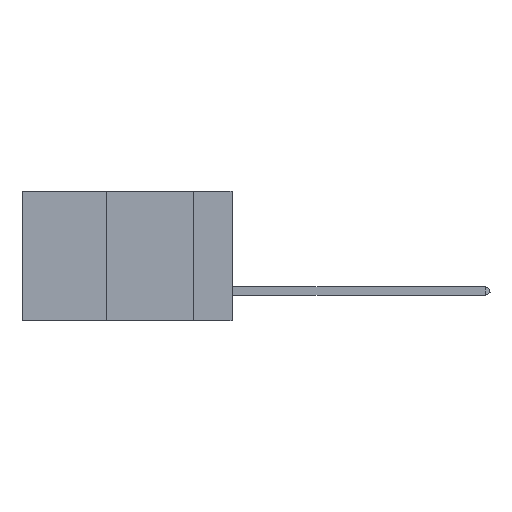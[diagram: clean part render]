
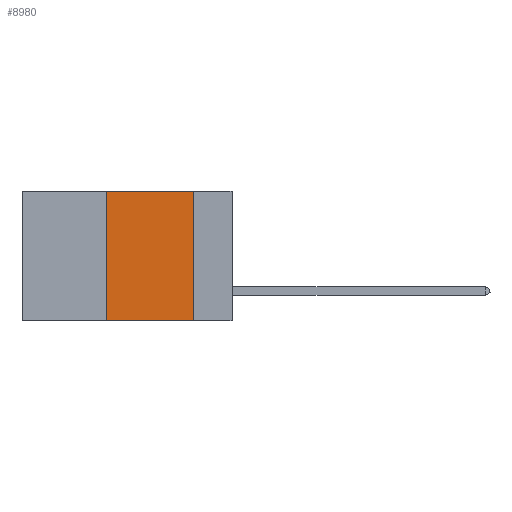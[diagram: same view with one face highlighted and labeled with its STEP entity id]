
A CAD part, left-side view. The second image highlights one B-rep face of the part: STEP entity #8980.
In plain terms, the highlighted planar face has unit normal (-1, 0, 0).
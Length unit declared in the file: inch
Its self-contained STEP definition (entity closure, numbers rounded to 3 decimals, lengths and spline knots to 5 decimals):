
#90 = VERTEX_POINT ( 'NONE', #13206 ) ;
#434 = CARTESIAN_POINT ( 'NONE',  ( 0., 0.6, -0.37 ) ) ;
#2119 = VECTOR ( 'NONE', #6401, 39.37008 ) ;
#2528 = VECTOR ( 'NONE', #12863, 39.37008 ) ;
#2623 = LINE ( 'NONE', #9049, #10432 ) ;
#2697 = LINE ( 'NONE', #4594, #2528 ) ;
#4179 = CARTESIAN_POINT ( 'NONE',  ( 0., 0.36, -0.37 ) ) ;
#4324 = CARTESIAN_POINT ( 'NONE',  ( 0., 0.36, 0. ) ) ;
#4594 = CARTESIAN_POINT ( 'NONE',  ( 0., 0.36, 0. ) ) ;
#4645 = PLANE ( 'NONE',  #12801 ) ;
#4798 = CARTESIAN_POINT ( 'NONE',  ( 0., 0.6, 0. ) ) ;
#5038 = EDGE_CURVE ( 'NONE', #10226, #90, #9944, .T. ) ;
#5310 = LINE ( 'NONE', #434, #12380 ) ;
#5773 = DIRECTION ( 'NONE',  ( 0., 0., -1. ) ) ;
#6103 = VERTEX_POINT ( 'NONE', #6731 ) ;
#6310 = EDGE_CURVE ( 'NONE', #90, #6103, #2623, .T. ) ;
#6401 = DIRECTION ( 'NONE',  ( 0., -1., 0. ) ) ;
#6731 = CARTESIAN_POINT ( 'NONE',  ( 0., 0.11, -0.37 ) ) ;
#7592 = DIRECTION ( 'NONE',  ( 0., 0., -1. ) ) ;
#8919 = ORIENTED_EDGE ( 'NONE', *, *, #6310, .F. ) ;
#8961 = EDGE_CURVE ( 'NONE', #11784, #10226, #2697, .T. ) ;
#8980 = ADVANCED_FACE ( 'NONE', ( #14331 ), #4645, .F. ) ;
#9049 = CARTESIAN_POINT ( 'NONE',  ( 0., 0.11, 0. ) ) ;
#9664 = ORIENTED_EDGE ( 'NONE', *, *, #13613, .T. ) ;
#9710 = EDGE_LOOP ( 'NONE', ( #8919, #13636, #14198, #9664 ) ) ;
#9944 = LINE ( 'NONE', #11164, #2119 ) ;
#10226 = VERTEX_POINT ( 'NONE', #4324 ) ;
#10432 = VECTOR ( 'NONE', #7592, 39.37008 ) ;
#11164 = CARTESIAN_POINT ( 'NONE',  ( 0., 0.6, 0. ) ) ;
#11644 = DIRECTION ( 'NONE',  ( 0., -1., 0. ) ) ;
#11784 = VERTEX_POINT ( 'NONE', #4179 ) ;
#12380 = VECTOR ( 'NONE', #11644, 39.37008 ) ;
#12801 = AXIS2_PLACEMENT_3D ( 'NONE', #4798, #13891, #5773 ) ;
#12863 = DIRECTION ( 'NONE',  ( 0., 0., 1. ) ) ;
#13206 = CARTESIAN_POINT ( 'NONE',  ( 0., 0.11, 0. ) ) ;
#13613 = EDGE_CURVE ( 'NONE', #11784, #6103, #5310, .T. ) ;
#13636 = ORIENTED_EDGE ( 'NONE', *, *, #5038, .F. ) ;
#13891 = DIRECTION ( 'NONE',  ( 1., 0., 0. ) ) ;
#14198 = ORIENTED_EDGE ( 'NONE', *, *, #8961, .F. ) ;
#14331 = FACE_OUTER_BOUND ( 'NONE', #9710, .T. ) ;
